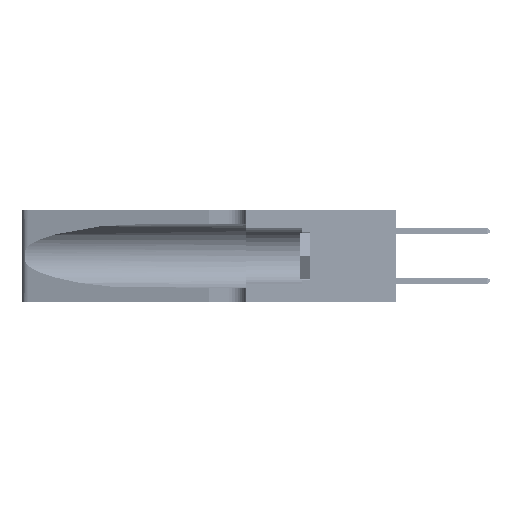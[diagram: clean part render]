
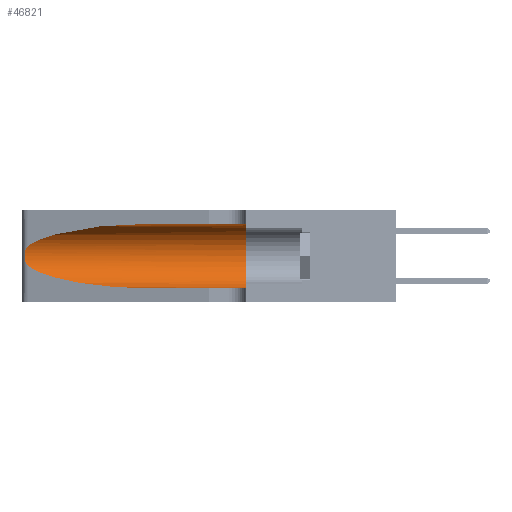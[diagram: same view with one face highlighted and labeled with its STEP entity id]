
A CAD part, left-side view. The second image highlights one B-rep face of the part: STEP entity #46821.
In plain terms, the highlighted cylindrical face has radius 3.308 mm (diameter 6.617 mm), a partial arc.
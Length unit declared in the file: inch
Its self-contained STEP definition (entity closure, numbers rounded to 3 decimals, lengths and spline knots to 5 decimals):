
#43 = ORIENTED_EDGE ( 'NONE', *, *, #15398, .T. ) ;
#88 = VERTEX_POINT ( 'NONE', #18073 ) ;
#224 = CARTESIAN_POINT ( 'NONE',  ( 0.25555, 1.22993, 0.14849 ) ) ;
#622 = CARTESIAN_POINT ( 'NONE',  ( 0.18966, 0.96281, 0.31525 ) ) ;
#902 = CARTESIAN_POINT ( 'NONE',  ( 0.25555, 1.22994, 0.2215 ) ) ;
#1453 = CARTESIAN_POINT ( 'NONE',  ( 0.18966, 0.96281, 0.05475 ) ) ;
#3124 = EDGE_CURVE ( 'NONE', #20689, #20713, #43058, .T. ) ;
#3320 = EDGE_LOOP ( 'NONE', ( #44833, #43, #33740, #49098, #29716, #33912 ) ) ;
#4242 = CARTESIAN_POINT ( 'NONE',  ( 0.25487, 1.22718, 0.22369 ) ) ;
#4331 = CARTESIAN_POINT ( 'NONE',  ( 0.1305, 0.72297, 0.31525 ) ) ;
#5155 = CARTESIAN_POINT ( 'NONE',  ( 0.25487, 1.22718, 0.14631 ) ) ;
#8488 = CARTESIAN_POINT ( 'NONE',  ( 0.25787, 1.23484, 0.2124 ) ) ;
#8996 = CARTESIAN_POINT ( 'NONE',  ( 0.26018, 1.23835, 0.19895 ) ) ;
#9761 = VERTEX_POINT ( 'NONE', #4242 ) ;
#10396 = VECTOR ( 'NONE', #35665, 39.37008 ) ;
#11897 = CARTESIAN_POINT ( 'NONE',  ( 0.1305, 0.35, 0.05475 ) ) ;
#12593 = CARTESIAN_POINT ( 'NONE',  ( 0.1305, 0.72297, 0.05475 ) ) ;
#13031 = CARTESIAN_POINT ( 'NONE',  ( 0.25854, 1.2359, 0.20912 ) ) ;
#14189 = CARTESIAN_POINT ( 'NONE',  ( 0.1305, 0.35, 0.185 ) ) ;
#14479 = AXIS2_PLACEMENT_3D ( 'NONE', #25215, #41178, #17262 ) ;
#15398 = EDGE_CURVE ( 'NONE', #9761, #33361, #45606, .T. ) ;
#16712 = CARTESIAN_POINT ( 'NONE',  ( 0.25639, 1.23186, 0.15144 ) ) ;
#17059 = CARTESIAN_POINT ( 'NONE',  ( 0.26075, 1.23896, 0.178 ) ) ;
#17262 = DIRECTION ( 'NONE',  ( 0., 0., -1. ) ) ;
#18073 = CARTESIAN_POINT ( 'NONE',  ( 0.1305, 0.35, 0.31525 ) ) ;
#20689 = VERTEX_POINT ( 'NONE', #12593 ) ;
#20713 = VERTEX_POINT ( 'NONE', #11897 ) ;
#23417 = EDGE_CURVE ( 'NONE', #40037, #88, #31752, .T. ) ;
#23538 = CARTESIAN_POINT ( 'NONE',  ( 0.1305, 1.61858, 0.31525 ) ) ;
#24657 = CARTESIAN_POINT ( 'NONE',  ( 0.25789, 1.23486, 0.15765 ) ) ;
#25215 = CARTESIAN_POINT ( 'NONE',  ( 0.1305, 1.61858, 0.185 ) ) ;
#28554 = CARTESIAN_POINT ( 'NONE',  ( 0.2373, 1.15595, 0.28018 ) ) ;
#28943 = CIRCLE ( 'NONE', #50547, 0.13025 ) ;
#28957 = EDGE_CURVE ( 'NONE', #40037, #9761, #46575, .T. ) ;
#29094 = DIRECTION ( 'NONE',  ( 0., 0., 1. ) ) ;
#29716 = ORIENTED_EDGE ( 'NONE', *, *, #50493, .F. ) ;
#31752 = LINE ( 'NONE', #23538, #10396 ) ;
#32863 = CARTESIAN_POINT ( 'NONE',  ( 0.1305, 1.61858, 0.05475 ) ) ;
#33050 =( BOUNDED_CURVE ( )  B_SPLINE_CURVE ( 3, ( #5155, #49232, #1453, #45206 ),
 .UNSPECIFIED., .F., .T. ) 
 B_SPLINE_CURVE_WITH_KNOTS ( ( 4, 4 ),
 ( 3.44316, 4.71239 ),
 .UNSPECIFIED. ) 
 CURVE ( )  GEOMETRIC_REPRESENTATION_ITEM ( )  RATIONAL_B_SPLINE_CURVE ( ( 1., 0.87, 0.87, 1. ) ) 
 REPRESENTATION_ITEM ( '' )  );
#33361 = VERTEX_POINT ( 'NONE', #48218 ) ;
#33653 = CYLINDRICAL_SURFACE ( 'NONE', #14479, 0.13025 ) ;
#33740 = ORIENTED_EDGE ( 'NONE', *, *, #48784, .T. ) ;
#33912 = ORIENTED_EDGE ( 'NONE', *, *, #23417, .F. ) ;
#35665 = DIRECTION ( 'NONE',  ( 0., -1., 0. ) ) ;
#36185 = FACE_OUTER_BOUND ( 'NONE', #3320, .T. ) ;
#36469 = CARTESIAN_POINT ( 'NONE',  ( 0.25487, 1.22718, 0.22369 ) ) ;
#36598 = CARTESIAN_POINT ( 'NONE',  ( 0.25487, 1.22718, 0.22369 ) ) ;
#36753 = DIRECTION ( 'NONE',  ( 0., -1., 0. ) ) ;
#37111 = CARTESIAN_POINT ( 'NONE',  ( 0.25639, 1.23184, 0.21858 ) ) ;
#40037 = VERTEX_POINT ( 'NONE', #43324 ) ;
#40453 = CARTESIAN_POINT ( 'NONE',  ( 0.26075, 1.23896, 0.19203 ) ) ;
#40624 = CARTESIAN_POINT ( 'NONE',  ( 0.26017, 1.23833, 0.17102 ) ) ;
#41178 = DIRECTION ( 'NONE',  ( 0., -1., 0. ) ) ;
#43058 = LINE ( 'NONE', #32863, #48081 ) ;
#43324 = CARTESIAN_POINT ( 'NONE',  ( 0.1305, 0.72297, 0.31525 ) ) ;
#44833 = ORIENTED_EDGE ( 'NONE', *, *, #28957, .T. ) ;
#44835 = CARTESIAN_POINT ( 'NONE',  ( 0.25487, 1.22718, 0.14631 ) ) ;
#45206 = CARTESIAN_POINT ( 'NONE',  ( 0.1305, 0.72297, 0.05475 ) ) ;
#45606 = B_SPLINE_CURVE_WITH_KNOTS ( 'NONE', 3,
 ( #36598, #902, #37111, #8488, #13031, #8996, #40453, #17059, #40624, #48694, #24657, #16712, #224, #44835 ),
 .UNSPECIFIED., .F., .F.,
 ( 4, 2, 2, 2, 2, 2, 4 ),
 ( 0., 0.00027, 0.00053, 0.00107, 0.0016, 0.00187, 0.00214 ),
 .UNSPECIFIED. ) ;
#46575 =( BOUNDED_CURVE ( )  B_SPLINE_CURVE ( 3, ( #4331, #622, #28554, #36469 ),
 .UNSPECIFIED., .F., .F. ) 
 B_SPLINE_CURVE_WITH_KNOTS ( ( 4, 4 ),
 ( 1.5708, 2.84003 ),
 .UNSPECIFIED. ) 
 CURVE ( )  GEOMETRIC_REPRESENTATION_ITEM ( )  RATIONAL_B_SPLINE_CURVE ( ( 1., 0.87, 0.87, 1. ) ) 
 REPRESENTATION_ITEM ( '' )  );
#46821 = ADVANCED_FACE ( 'NONE', ( #36185 ), #33653, .F. ) ;
#48081 = VECTOR ( 'NONE', #36753, 39.37008 ) ;
#48218 = CARTESIAN_POINT ( 'NONE',  ( 0.25487, 1.22718, 0.14631 ) ) ;
#48694 = CARTESIAN_POINT ( 'NONE',  ( 0.25856, 1.23593, 0.16098 ) ) ;
#48784 = EDGE_CURVE ( 'NONE', #33361, #20689, #33050, .T. ) ;
#49098 = ORIENTED_EDGE ( 'NONE', *, *, #3124, .T. ) ;
#49232 = CARTESIAN_POINT ( 'NONE',  ( 0.2373, 1.15595, 0.08982 ) ) ;
#49453 = DIRECTION ( 'NONE',  ( 0., 1., 0. ) ) ;
#50493 = EDGE_CURVE ( 'NONE', #88, #20713, #28943, .T. ) ;
#50547 = AXIS2_PLACEMENT_3D ( 'NONE', #14189, #49453, #29094 ) ;
